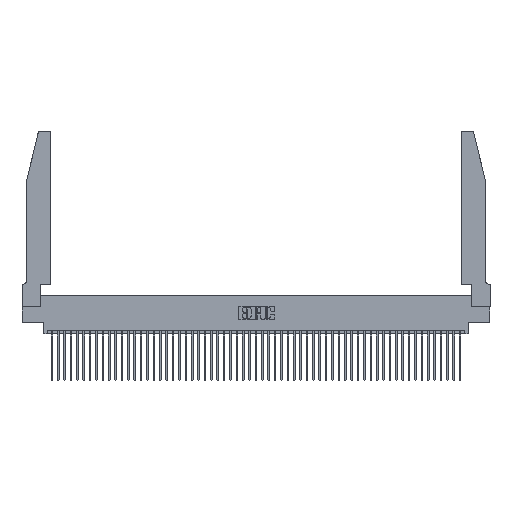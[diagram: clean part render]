
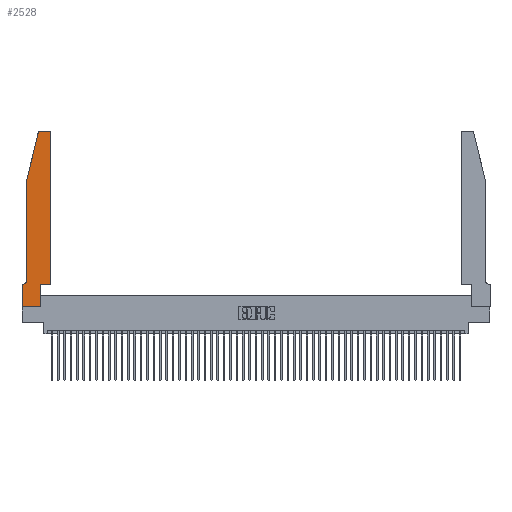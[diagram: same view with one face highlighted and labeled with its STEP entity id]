
A CAD part, top view. The second image highlights one B-rep face of the part: STEP entity #2528.
In plain terms, the highlighted planar face has unit normal (0, 0, 1).
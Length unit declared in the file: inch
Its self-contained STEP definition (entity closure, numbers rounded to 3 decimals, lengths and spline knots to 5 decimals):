
#1792 = EDGE_CURVE ( 'NONE', #23400, #16561, #20468, .T. ) ;
#2165 = LINE ( 'NONE', #20995, #43028 ) ;
#2453 = ORIENTED_EDGE ( 'NONE', *, *, #50602, .T. ) ;
#2497 = DIRECTION ( 'NONE',  ( 0., 0., -1. ) ) ;
#2522 = VERTEX_POINT ( 'NONE', #51952 ) ;
#2528 = ADVANCED_FACE ( 'NONE', ( #10070 ), #3195, .T. ) ;
#2695 = CARTESIAN_POINT ( 'NONE',  ( 0.2605, 2.75, 0.37 ) ) ;
#2932 = DIRECTION ( 'NONE',  ( 1., 0., 0. ) ) ;
#3192 = CARTESIAN_POINT ( 'NONE',  ( 0.0055, 0.35, 0.37 ) ) ;
#3195 = PLANE ( 'NONE',  #4024 ) ;
#3730 = EDGE_CURVE ( 'NONE', #52327, #29277, #2165, .T. ) ;
#4024 = AXIS2_PLACEMENT_3D ( 'NONE', #7380, #35838, #11486 ) ;
#4418 = ORIENTED_EDGE ( 'NONE', *, *, #5085, .T. ) ;
#4660 = DIRECTION ( 'NONE',  ( 0., -1., 0. ) ) ;
#4891 = ORIENTED_EDGE ( 'NONE', *, *, #24937, .T. ) ;
#5026 = ORIENTED_EDGE ( 'NONE', *, *, #16838, .T. ) ;
#5070 = DIRECTION ( 'NONE',  ( -1., 0., 0. ) ) ;
#5085 = EDGE_CURVE ( 'NONE', #45191, #33676, #48166, .T. ) ;
#6266 = VERTEX_POINT ( 'NONE', #15912 ) ;
#6463 = CARTESIAN_POINT ( 'NONE',  ( 0.4205, 2.75, 0.37 ) ) ;
#6851 = ORIENTED_EDGE ( 'NONE', *, *, #1792, .T. ) ;
#7380 = CARTESIAN_POINT ( 'NONE',  ( 0., 0.35, 0.37 ) ) ;
#8354 = ORIENTED_EDGE ( 'NONE', *, *, #43150, .T. ) ;
#8505 = EDGE_CURVE ( 'NONE', #31312, #23400, #49669, .T. ) ;
#8646 = EDGE_CURVE ( 'NONE', #49406, #31312, #33836, .T. ) ;
#8915 = DIRECTION ( 'NONE',  ( 0., 0., 1. ) ) ;
#9281 = LINE ( 'NONE', #19764, #52481 ) ;
#10070 = FACE_OUTER_BOUND ( 'NONE', #30501, .T. ) ;
#11486 = DIRECTION ( 'NONE',  ( 1., 0., 0. ) ) ;
#12214 = VECTOR ( 'NONE', #47586, 39.37008 ) ;
#12862 = CARTESIAN_POINT ( 'NONE',  ( 0.4505, 2.72, 0.37 ) ) ;
#13204 = AXIS2_PLACEMENT_3D ( 'NONE', #38066, #13722, #42130 ) ;
#13722 = DIRECTION ( 'NONE',  ( 0., 0., 1. ) ) ;
#14343 = CARTESIAN_POINT ( 'NONE',  ( 0.0755, 2., 0.37 ) ) ;
#15351 = LINE ( 'NONE', #15459, #46432 ) ;
#15459 = CARTESIAN_POINT ( 'NONE',  ( 0.2865, 0.35, 0.37 ) ) ;
#15912 = CARTESIAN_POINT ( 'NONE',  ( 0.2865, 0., 0.37 ) ) ;
#16220 = CARTESIAN_POINT ( 'NONE',  ( 0., 0., 0.37 ) ) ;
#16561 = VERTEX_POINT ( 'NONE', #49533 ) ;
#16838 = EDGE_CURVE ( 'NONE', #29277, #45191, #38448, .T. ) ;
#16904 = CARTESIAN_POINT ( 'NONE',  ( 0., 0.35, 0.37 ) ) ;
#17138 = CARTESIAN_POINT ( 'NONE',  ( 0.0755, 0.35, 0.37 ) ) ;
#17715 = ORIENTED_EDGE ( 'NONE', *, *, #3730, .T. ) ;
#18757 = EDGE_CURVE ( 'NONE', #39582, #6266, #9281, .T. ) ;
#19192 = VECTOR ( 'NONE', #27226, 39.37008 ) ;
#19256 = CARTESIAN_POINT ( 'NONE',  ( 0.4505, 0.35, 0.37 ) ) ;
#19351 = ORIENTED_EDGE ( 'NONE', *, *, #18757, .T. ) ;
#19590 = DIRECTION ( 'NONE',  ( 0., 1., 0. ) ) ;
#19764 = CARTESIAN_POINT ( 'NONE',  ( 0., 0., 0.37 ) ) ;
#20423 = ORIENTED_EDGE ( 'NONE', *, *, #39044, .T. ) ;
#20468 = LINE ( 'NONE', #2695, #19192 ) ;
#20604 = CARTESIAN_POINT ( 'NONE',  ( 0.2865, 0.35, 0.37 ) ) ;
#20995 = CARTESIAN_POINT ( 'NONE',  ( 0.0755, 2., 0.37 ) ) ;
#21005 = ORIENTED_EDGE ( 'NONE', *, *, #8505, .T. ) ;
#23400 = VERTEX_POINT ( 'NONE', #6463 ) ;
#23744 = CARTESIAN_POINT ( 'NONE',  ( 0.4505, 0.35, 0.37 ) ) ;
#24624 = CARTESIAN_POINT ( 'NONE',  ( 0.0755, 2., 0.37 ) ) ;
#24937 = EDGE_CURVE ( 'NONE', #33676, #39582, #41870, .T. ) ;
#27037 = CARTESIAN_POINT ( 'NONE',  ( 0.0055, 0.42, 0.37 ) ) ;
#27226 = DIRECTION ( 'NONE',  ( -1., 0., 0. ) ) ;
#27435 = CARTESIAN_POINT ( 'NONE',  ( 0.4505, 0.35, 0.37 ) ) ;
#28511 = VECTOR ( 'NONE', #49494, 39.37008 ) ;
#29277 = VERTEX_POINT ( 'NONE', #30154 ) ;
#29306 = CARTESIAN_POINT ( 'NONE',  ( 0., 0., 0.37 ) ) ;
#29728 = VERTEX_POINT ( 'NONE', #20604 ) ;
#30154 = CARTESIAN_POINT ( 'NONE',  ( 0.0755, 0.42, 0.37 ) ) ;
#30501 = EDGE_LOOP ( 'NONE', ( #6851, #20423, #2453, #17715, #5026, #4418, #4891, #19351, #8354, #45570, #30739, #21005 ) ) ;
#30739 = ORIENTED_EDGE ( 'NONE', *, *, #8646, .T. ) ;
#31131 = DIRECTION ( 'NONE',  ( -1., 0., 0. ) ) ;
#31312 = VERTEX_POINT ( 'NONE', #12862 ) ;
#32709 = EDGE_CURVE ( 'NONE', #29728, #49406, #48186, .T. ) ;
#33268 = CARTESIAN_POINT ( 'NONE',  ( 0.284, 2.72, 0.37 ) ) ;
#33676 = VERTEX_POINT ( 'NONE', #16904 ) ;
#33836 = LINE ( 'NONE', #19256, #12214 ) ;
#35838 = DIRECTION ( 'NONE',  ( 0., 0., 1. ) ) ;
#36227 = AXIS2_PLACEMENT_3D ( 'NONE', #27037, #2497, #31131 ) ;
#37373 = AXIS2_PLACEMENT_3D ( 'NONE', #33268, #8915, #37392 ) ;
#37392 = DIRECTION ( 'NONE',  ( 1., 0., 0. ) ) ;
#37439 = VECTOR ( 'NONE', #5070, 39.37008 ) ;
#38066 = CARTESIAN_POINT ( 'NONE',  ( 0.4205, 2.72, 0.37 ) ) ;
#38448 = CIRCLE ( 'NONE', #36227, 0.07 ) ;
#39044 = EDGE_CURVE ( 'NONE', #16561, #2522, #44142, .T. ) ;
#39582 = VERTEX_POINT ( 'NONE', #16220 ) ;
#41200 = VECTOR ( 'NONE', #42737, 39.37008 ) ;
#41870 = LINE ( 'NONE', #29306, #28511 ) ;
#42130 = DIRECTION ( 'NONE',  ( 1., 0., 0. ) ) ;
#42737 = DIRECTION ( 'NONE',  ( -0.239, -0.971, 0. ) ) ;
#43028 = VECTOR ( 'NONE', #4660, 39.37008 ) ;
#43150 = EDGE_CURVE ( 'NONE', #6266, #29728, #15351, .T. ) ;
#44142 = CIRCLE ( 'NONE', #37373, 0.03 ) ;
#45191 = VERTEX_POINT ( 'NONE', #3192 ) ;
#45570 = ORIENTED_EDGE ( 'NONE', *, *, #32709, .T. ) ;
#46432 = VECTOR ( 'NONE', #19590, 39.37008 ) ;
#46937 = VECTOR ( 'NONE', #2932, 39.37008 ) ;
#47586 = DIRECTION ( 'NONE',  ( 0., 1., 0. ) ) ;
#48049 = DIRECTION ( 'NONE',  ( 1., 0., 0. ) ) ;
#48166 = LINE ( 'NONE', #17138, #37439 ) ;
#48186 = LINE ( 'NONE', #27435, #46937 ) ;
#49406 = VERTEX_POINT ( 'NONE', #23744 ) ;
#49494 = DIRECTION ( 'NONE',  ( 0., -1., 0. ) ) ;
#49533 = CARTESIAN_POINT ( 'NONE',  ( 0.284, 2.75, 0.37 ) ) ;
#49669 = CIRCLE ( 'NONE', #13204, 0.03 ) ;
#50602 = EDGE_CURVE ( 'NONE', #2522, #52327, #50644, .T. ) ;
#50644 = LINE ( 'NONE', #14343, #41200 ) ;
#51952 = CARTESIAN_POINT ( 'NONE',  ( 0.25487, 2.72718, 0.37 ) ) ;
#52327 = VERTEX_POINT ( 'NONE', #24624 ) ;
#52481 = VECTOR ( 'NONE', #48049, 39.37008 ) ;
